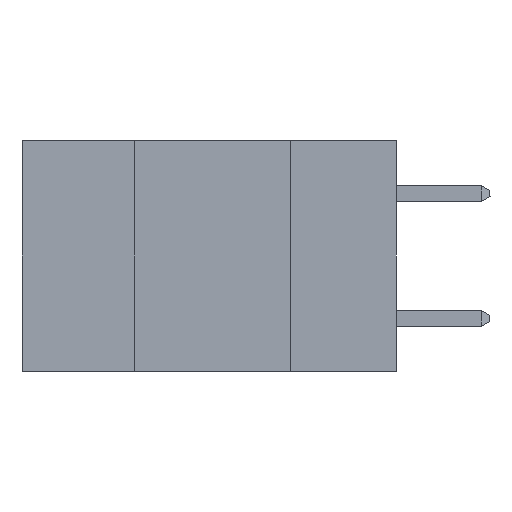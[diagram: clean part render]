
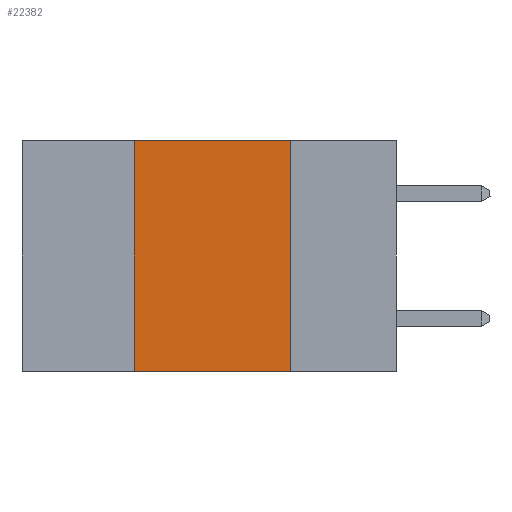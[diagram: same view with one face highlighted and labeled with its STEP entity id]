
A CAD part, left-side view. The second image highlights one B-rep face of the part: STEP entity #22382.
In plain terms, the highlighted planar face has unit normal (-1, 0, 0).
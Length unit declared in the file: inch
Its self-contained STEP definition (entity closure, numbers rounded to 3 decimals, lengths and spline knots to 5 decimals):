
#575 = AXIS2_PLACEMENT_3D ( 'NONE', #16693, #18400, #8101 ) ;
#1833 = VECTOR ( 'NONE', #18916, 39.37008 ) ;
#2020 = LINE ( 'NONE', #19055, #6139 ) ;
#2659 = CARTESIAN_POINT ( 'NONE',  ( 0., 0.42, 0. ) ) ;
#2864 = VECTOR ( 'NONE', #8065, 39.37008 ) ;
#3699 = ORIENTED_EDGE ( 'NONE', *, *, #9715, .F. ) ;
#4550 = CARTESIAN_POINT ( 'NONE',  ( 0., 0.42, -0.37 ) ) ;
#4589 = PLANE ( 'NONE',  #575 ) ;
#4819 = LINE ( 'NONE', #6423, #13456 ) ;
#6139 = VECTOR ( 'NONE', #20838, 39.37008 ) ;
#6419 = ORIENTED_EDGE ( 'NONE', *, *, #16507, .F. ) ;
#6423 = CARTESIAN_POINT ( 'NONE',  ( 0., 0.17, -0.37 ) ) ;
#7159 = ORIENTED_EDGE ( 'NONE', *, *, #21408, .F. ) ;
#8065 = DIRECTION ( 'NONE',  ( 0., -1., 0. ) ) ;
#8101 = DIRECTION ( 'NONE',  ( 0., 0., -1. ) ) ;
#8187 = DIRECTION ( 'NONE',  ( 0., 0., -1. ) ) ;
#8493 = CARTESIAN_POINT ( 'NONE',  ( 0., 0.17, -0.37 ) ) ;
#9715 = EDGE_CURVE ( 'NONE', #17649, #10617, #20786, .T. ) ;
#9990 = EDGE_CURVE ( 'NONE', #12447, #10636, #2020, .T. ) ;
#10558 = LINE ( 'NONE', #17172, #1833 ) ;
#10617 = VERTEX_POINT ( 'NONE', #18725 ) ;
#10631 = EDGE_LOOP ( 'NONE', ( #6419, #3699, #7159, #11971 ) ) ;
#10636 = VERTEX_POINT ( 'NONE', #8493 ) ;
#11971 = ORIENTED_EDGE ( 'NONE', *, *, #9990, .T. ) ;
#12447 = VERTEX_POINT ( 'NONE', #4550 ) ;
#13456 = VECTOR ( 'NONE', #8187, 39.37008 ) ;
#15899 = FACE_OUTER_BOUND ( 'NONE', #10631, .T. ) ;
#16507 = EDGE_CURVE ( 'NONE', #10617, #10636, #4819, .T. ) ;
#16693 = CARTESIAN_POINT ( 'NONE',  ( 0., 0.6, 0. ) ) ;
#17172 = CARTESIAN_POINT ( 'NONE',  ( 0., 0.42, -0.37 ) ) ;
#17649 = VERTEX_POINT ( 'NONE', #2659 ) ;
#18367 = CARTESIAN_POINT ( 'NONE',  ( 0., 0.6, 0. ) ) ;
#18400 = DIRECTION ( 'NONE',  ( 1., 0., 0. ) ) ;
#18725 = CARTESIAN_POINT ( 'NONE',  ( 0., 0.17, 0. ) ) ;
#18916 = DIRECTION ( 'NONE',  ( 0., 0., 1. ) ) ;
#19055 = CARTESIAN_POINT ( 'NONE',  ( 0., 0.6, -0.37 ) ) ;
#20786 = LINE ( 'NONE', #18367, #2864 ) ;
#20838 = DIRECTION ( 'NONE',  ( 0., -1., 0. ) ) ;
#21408 = EDGE_CURVE ( 'NONE', #12447, #17649, #10558, .T. ) ;
#22382 = ADVANCED_FACE ( 'NONE', ( #15899 ), #4589, .F. ) ;
